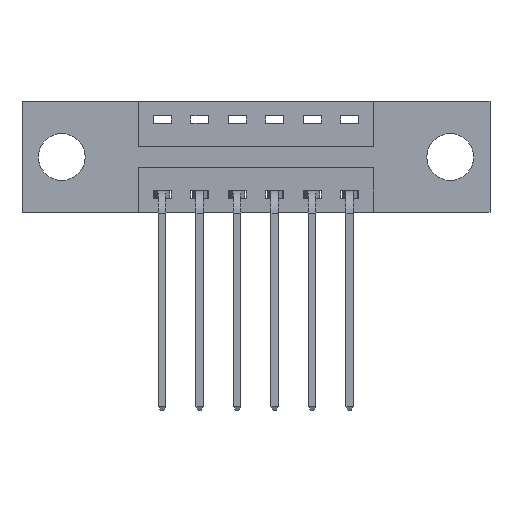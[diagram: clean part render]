
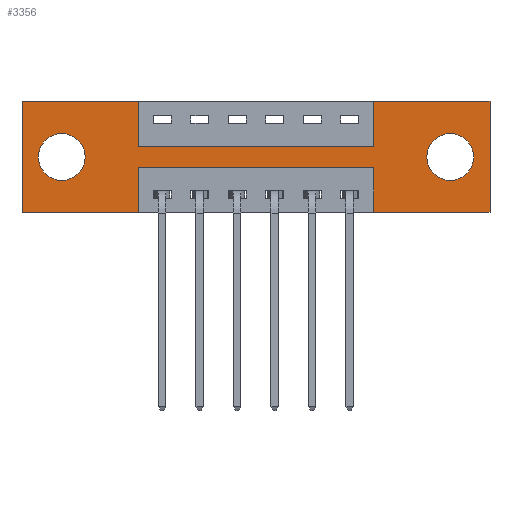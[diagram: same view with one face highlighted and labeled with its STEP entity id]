
A CAD part, front view. The second image highlights one B-rep face of the part: STEP entity #3356.
In plain terms, the highlighted planar face has unit normal (0, -1, 0).
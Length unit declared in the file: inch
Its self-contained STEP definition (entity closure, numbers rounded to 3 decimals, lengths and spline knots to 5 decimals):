
#30 = ORIENTED_EDGE ( 'NONE', *, *, #5984, .F. ) ;
#31 = ORIENTED_EDGE ( 'NONE', *, *, #4455, .F. ) ;
#141 = VECTOR ( 'NONE', #4041, 39.37008 ) ;
#193 = ORIENTED_EDGE ( 'NONE', *, *, #3496, .F. ) ;
#207 = DIRECTION ( 'NONE',  ( 0., 0., 1. ) ) ;
#309 = ORIENTED_EDGE ( 'NONE', *, *, #4650, .F. ) ;
#313 = ORIENTED_EDGE ( 'NONE', *, *, #3707, .F. ) ;
#336 = ORIENTED_EDGE ( 'NONE', *, *, #397, .T. ) ;
#370 = EDGE_CURVE ( 'NONE', #3757, #5551, #3655, .T. ) ;
#371 = CARTESIAN_POINT ( 'NONE',  ( 0.1325, 0., -0.185 ) ) ;
#372 = DIRECTION ( 'NONE',  ( 0., 1., 0. ) ) ;
#384 = VERTEX_POINT ( 'NONE', #1782 ) ;
#387 = CIRCLE ( 'NONE', #4129, 0.078 ) ;
#397 = EDGE_CURVE ( 'NONE', #384, #4082, #3229, .T. ) ;
#448 = ORIENTED_EDGE ( 'NONE', *, *, #3589, .T. ) ;
#505 = CARTESIAN_POINT ( 'NONE',  ( 1.4275, 0., -0.185 ) ) ;
#537 = CARTESIAN_POINT ( 'NONE',  ( 1.1725, 0., -0.15 ) ) ;
#550 = ORIENTED_EDGE ( 'NONE', *, *, #3487, .F. ) ;
#557 = ORIENTED_EDGE ( 'NONE', *, *, #8264, .F. ) ;
#595 = ORIENTED_EDGE ( 'NONE', *, *, #7580, .T. ) ;
#609 = VERTEX_POINT ( 'NONE', #7326 ) ;
#803 = VECTOR ( 'NONE', #1955, 39.37008 ) ;
#830 = LINE ( 'NONE', #2008, #803 ) ;
#1073 = DIRECTION ( 'NONE',  ( 0., 0., 1. ) ) ;
#1096 = CARTESIAN_POINT ( 'NONE',  ( 1.4275, 0., -0.185 ) ) ;
#1204 = DIRECTION ( 'NONE',  ( 0., 0., -1. ) ) ;
#1338 = ORIENTED_EDGE ( 'NONE', *, *, #7686, .T. ) ;
#1348 = VECTOR ( 'NONE', #3473, 39.37008 ) ;
#1367 = VERTEX_POINT ( 'NONE', #2054 ) ;
#1406 = ORIENTED_EDGE ( 'NONE', *, *, #2840, .F. ) ;
#1782 = CARTESIAN_POINT ( 'NONE',  ( 1.4275, 0., -0.107 ) ) ;
#1879 = CARTESIAN_POINT ( 'NONE',  ( 1.56, 0., -0.37 ) ) ;
#1939 = VECTOR ( 'NONE', #8502, 39.37008 ) ;
#1955 = DIRECTION ( 'NONE',  ( 0., 0., -1. ) ) ;
#1968 = ORIENTED_EDGE ( 'NONE', *, *, #8548, .F. ) ;
#1989 = CARTESIAN_POINT ( 'NONE',  ( 0.3875, 0., -0.22 ) ) ;
#2008 = CARTESIAN_POINT ( 'NONE',  ( 0.3875, 0., 0. ) ) ;
#2021 = CARTESIAN_POINT ( 'NONE',  ( 0.3875, 0., 0. ) ) ;
#2054 = CARTESIAN_POINT ( 'NONE',  ( 0.3875, 0., -0.15 ) ) ;
#2375 = DIRECTION ( 'NONE',  ( 0., 0., -1. ) ) ;
#2406 = LINE ( 'NONE', #8352, #2503 ) ;
#2503 = VECTOR ( 'NONE', #8283, 39.37008 ) ;
#2591 = DIRECTION ( 'NONE',  ( 0., 0., 1. ) ) ;
#2624 = CARTESIAN_POINT ( 'NONE',  ( 1.1725, 0., 0. ) ) ;
#2656 = CARTESIAN_POINT ( 'NONE',  ( 1.56, 0., 0. ) ) ;
#2714 = AXIS2_PLACEMENT_3D ( 'NONE', #371, #372, #207 ) ;
#2739 = CARTESIAN_POINT ( 'NONE',  ( 1.1725, 0., 0. ) ) ;
#2787 = LINE ( 'NONE', #8360, #3251 ) ;
#2840 = EDGE_CURVE ( 'NONE', #609, #4658, #5329, .T. ) ;
#2842 = CARTESIAN_POINT ( 'NONE',  ( 1.4275, 0., -0.263 ) ) ;
#2921 = VERTEX_POINT ( 'NONE', #6718 ) ;
#2974 = CIRCLE ( 'NONE', #2714, 0.078 ) ;
#3018 = LINE ( 'NONE', #3971, #141 ) ;
#3059 = CARTESIAN_POINT ( 'NONE',  ( 0., 0., -0.37 ) ) ;
#3111 = DIRECTION ( 'NONE',  ( -1., 0., 0. ) ) ;
#3179 = VECTOR ( 'NONE', #3593, 39.37008 ) ;
#3229 = CIRCLE ( 'NONE', #8184, 0.078 ) ;
#3251 = VECTOR ( 'NONE', #6504, 39.37008 ) ;
#3356 = ADVANCED_FACE ( 'NONE', ( #7322, #6619, #6876 ), #5819, .T. ) ;
#3437 = CARTESIAN_POINT ( 'NONE',  ( 0., 0., 0. ) ) ;
#3473 = DIRECTION ( 'NONE',  ( 1., 0., 0. ) ) ;
#3487 = EDGE_CURVE ( 'NONE', #7636, #7612, #5282, .T. ) ;
#3496 = EDGE_CURVE ( 'NONE', #7914, #7541, #4854, .T. ) ;
#3517 = VECTOR ( 'NONE', #3111, 39.37008 ) ;
#3535 = CARTESIAN_POINT ( 'NONE',  ( 0., 0., 0. ) ) ;
#3589 = EDGE_CURVE ( 'NONE', #6708, #2921, #2974, .T. ) ;
#3593 = DIRECTION ( 'NONE',  ( -1., 0., 0. ) ) ;
#3648 = AXIS2_PLACEMENT_3D ( 'NONE', #505, #5495, #1204 ) ;
#3655 = LINE ( 'NONE', #4393, #3179 ) ;
#3707 = EDGE_CURVE ( 'NONE', #1367, #7636, #2406, .T. ) ;
#3757 = VERTEX_POINT ( 'NONE', #8095 ) ;
#3971 = CARTESIAN_POINT ( 'NONE',  ( 0.3875, 0., -0.37 ) ) ;
#4041 = DIRECTION ( 'NONE',  ( 0., 0., -1. ) ) ;
#4082 = VERTEX_POINT ( 'NONE', #2842 ) ;
#4129 = AXIS2_PLACEMENT_3D ( 'NONE', #4246, #8584, #4900 ) ;
#4246 = CARTESIAN_POINT ( 'NONE',  ( 0.1325, 0., -0.185 ) ) ;
#4298 = EDGE_CURVE ( 'NONE', #4658, #3757, #3018, .T. ) ;
#4384 = CARTESIAN_POINT ( 'NONE',  ( 1.1725, 0., -0.37 ) ) ;
#4393 = CARTESIAN_POINT ( 'NONE',  ( 0., 0., -0.37 ) ) ;
#4455 = EDGE_CURVE ( 'NONE', #7541, #7832, #4681, .T. ) ;
#4650 = EDGE_CURVE ( 'NONE', #5342, #1367, #830, .T. ) ;
#4656 = CIRCLE ( 'NONE', #3648, 0.078 ) ;
#4658 = VERTEX_POINT ( 'NONE', #1989 ) ;
#4681 = LINE ( 'NONE', #3059, #3517 ) ;
#4854 = LINE ( 'NONE', #2656, #4992 ) ;
#4872 = DIRECTION ( 'NONE',  ( 0., 1., 0. ) ) ;
#4900 = DIRECTION ( 'NONE',  ( 0., 0., 1. ) ) ;
#4992 = VECTOR ( 'NONE', #2375, 39.37008 ) ;
#5036 = CARTESIAN_POINT ( 'NONE',  ( 0., 0., -0.37 ) ) ;
#5075 = VECTOR ( 'NONE', #2591, 39.37008 ) ;
#5175 = EDGE_LOOP ( 'NONE', ( #6369, #1406, #30, #31, #193, #557, #550, #313, #309, #6566, #1968, #8261 ) ) ;
#5282 = LINE ( 'NONE', #2624, #5075 ) ;
#5329 = LINE ( 'NONE', #7938, #1939 ) ;
#5342 = VERTEX_POINT ( 'NONE', #2021 ) ;
#5351 = DIRECTION ( 'NONE',  ( 0., 0., -1. ) ) ;
#5495 = DIRECTION ( 'NONE',  ( 0., 1., 0. ) ) ;
#5551 = VERTEX_POINT ( 'NONE', #5036 ) ;
#5768 = DIRECTION ( 'NONE',  ( 0., 0., -1. ) ) ;
#5819 = PLANE ( 'NONE',  #8241 ) ;
#5898 = EDGE_CURVE ( 'NONE', #8329, #5342, #8097, .T. ) ;
#5946 = CARTESIAN_POINT ( 'NONE',  ( 0., 0., 0. ) ) ;
#5984 = EDGE_CURVE ( 'NONE', #7832, #609, #7372, .T. ) ;
#6003 = CARTESIAN_POINT ( 'NONE',  ( 0., 0., -0.37 ) ) ;
#6103 = DIRECTION ( 'NONE',  ( 0., -1., 0. ) ) ;
#6362 = CARTESIAN_POINT ( 'NONE',  ( 1.56, 0., 0. ) ) ;
#6369 = ORIENTED_EDGE ( 'NONE', *, *, #4298, .F. ) ;
#6504 = DIRECTION ( 'NONE',  ( 0., 0., 1. ) ) ;
#6538 = DIRECTION ( 'NONE',  ( 1., 0., 0. ) ) ;
#6566 = ORIENTED_EDGE ( 'NONE', *, *, #5898, .F. ) ;
#6619 = FACE_BOUND ( 'NONE', #8306, .T. ) ;
#6634 = EDGE_LOOP ( 'NONE', ( #336, #595 ) ) ;
#6641 = LINE ( 'NONE', #3437, #1348 ) ;
#6708 = VERTEX_POINT ( 'NONE', #7262 ) ;
#6718 = CARTESIAN_POINT ( 'NONE',  ( 0.1325, 0., -0.107 ) ) ;
#6876 = FACE_OUTER_BOUND ( 'NONE', #5175, .T. ) ;
#7262 = CARTESIAN_POINT ( 'NONE',  ( 0.1325, 0., -0.263 ) ) ;
#7322 = FACE_BOUND ( 'NONE', #6634, .T. ) ;
#7326 = CARTESIAN_POINT ( 'NONE',  ( 1.1725, 0., -0.22 ) ) ;
#7332 = VECTOR ( 'NONE', #1073, 39.37008 ) ;
#7372 = LINE ( 'NONE', #7843, #7332 ) ;
#7541 = VERTEX_POINT ( 'NONE', #1879 ) ;
#7580 = EDGE_CURVE ( 'NONE', #4082, #384, #4656, .T. ) ;
#7612 = VERTEX_POINT ( 'NONE', #2739 ) ;
#7636 = VERTEX_POINT ( 'NONE', #537 ) ;
#7686 = EDGE_CURVE ( 'NONE', #2921, #6708, #387, .T. ) ;
#7764 = VECTOR ( 'NONE', #6538, 39.37008 ) ;
#7832 = VERTEX_POINT ( 'NONE', #4384 ) ;
#7843 = CARTESIAN_POINT ( 'NONE',  ( 1.1725, 0., -0.37 ) ) ;
#7914 = VERTEX_POINT ( 'NONE', #6362 ) ;
#7938 = CARTESIAN_POINT ( 'NONE',  ( 0.3875, 0., -0.22 ) ) ;
#8095 = CARTESIAN_POINT ( 'NONE',  ( 0.3875, 0., -0.37 ) ) ;
#8097 = LINE ( 'NONE', #5946, #7764 ) ;
#8184 = AXIS2_PLACEMENT_3D ( 'NONE', #1096, #4872, #5351 ) ;
#8241 = AXIS2_PLACEMENT_3D ( 'NONE', #6003, #6103, #5768 ) ;
#8261 = ORIENTED_EDGE ( 'NONE', *, *, #370, .F. ) ;
#8264 = EDGE_CURVE ( 'NONE', #7612, #7914, #6641, .T. ) ;
#8283 = DIRECTION ( 'NONE',  ( 1., 0., 0. ) ) ;
#8306 = EDGE_LOOP ( 'NONE', ( #1338, #448 ) ) ;
#8329 = VERTEX_POINT ( 'NONE', #3535 ) ;
#8352 = CARTESIAN_POINT ( 'NONE',  ( 0.3875, 0., -0.15 ) ) ;
#8360 = CARTESIAN_POINT ( 'NONE',  ( 0., 0., 0. ) ) ;
#8502 = DIRECTION ( 'NONE',  ( -1., 0., 0. ) ) ;
#8548 = EDGE_CURVE ( 'NONE', #5551, #8329, #2787, .T. ) ;
#8584 = DIRECTION ( 'NONE',  ( 0., 1., 0. ) ) ;
